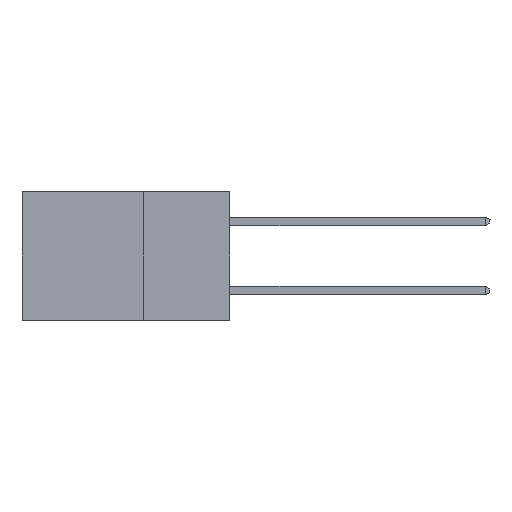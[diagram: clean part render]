
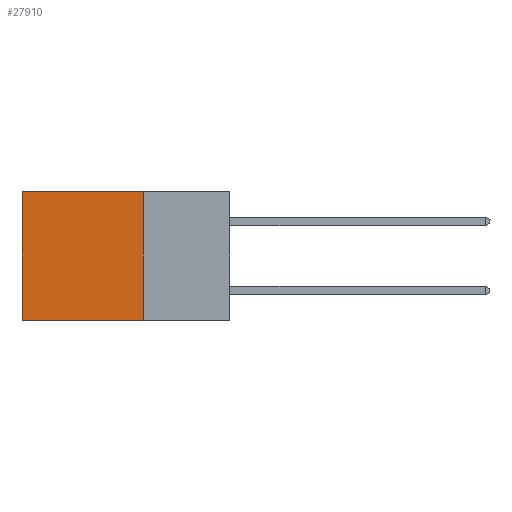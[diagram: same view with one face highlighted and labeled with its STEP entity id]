
A CAD part, left-side view. The second image highlights one B-rep face of the part: STEP entity #27910.
In plain terms, the highlighted planar face has unit normal (-1, 0, 0).
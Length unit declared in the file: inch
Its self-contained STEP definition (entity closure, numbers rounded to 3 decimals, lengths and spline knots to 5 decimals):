
#146 = VERTEX_POINT ( 'NONE', #16180 ) ;
#1535 = DIRECTION ( 'NONE',  ( 1., 0., 0. ) ) ;
#4924 = FACE_OUTER_BOUND ( 'NONE', #17492, .T. ) ;
#4960 = VECTOR ( 'NONE', #5991, 39.37008 ) ;
#5991 = DIRECTION ( 'NONE',  ( 0., 1., 0. ) ) ;
#7295 = DIRECTION ( 'NONE',  ( 0., 0., -1. ) ) ;
#7827 = CARTESIAN_POINT ( 'NONE',  ( 0.298, 0.6, 0. ) ) ;
#8591 = CARTESIAN_POINT ( 'NONE',  ( 0.298, 0.25, 0. ) ) ;
#10934 = CARTESIAN_POINT ( 'NONE',  ( 0.298, 0.25, -0.37 ) ) ;
#11558 = ORIENTED_EDGE ( 'NONE', *, *, #27721, .F. ) ;
#12032 = LINE ( 'NONE', #24882, #13230 ) ;
#12272 = VERTEX_POINT ( 'NONE', #10934 ) ;
#13230 = VECTOR ( 'NONE', #22468, 39.37008 ) ;
#13740 = VECTOR ( 'NONE', #7295, 39.37008 ) ;
#16180 = CARTESIAN_POINT ( 'NONE',  ( 0.298, 0.6, -0.37 ) ) ;
#16214 = EDGE_CURVE ( 'NONE', #20030, #17668, #18135, .T. ) ;
#16773 = PLANE ( 'NONE',  #28178 ) ;
#17492 = EDGE_LOOP ( 'NONE', ( #26882, #11558, #18700, #18011 ) ) ;
#17668 = VERTEX_POINT ( 'NONE', #7827 ) ;
#18011 = ORIENTED_EDGE ( 'NONE', *, *, #16214, .T. ) ;
#18135 = LINE ( 'NONE', #28933, #26448 ) ;
#18700 = ORIENTED_EDGE ( 'NONE', *, *, #28775, .F. ) ;
#19349 = DIRECTION ( 'NONE',  ( 0., 0., -1. ) ) ;
#19459 = CARTESIAN_POINT ( 'NONE',  ( 0.298, 0.25, 0. ) ) ;
#20030 = VERTEX_POINT ( 'NONE', #8591 ) ;
#20600 = LINE ( 'NONE', #23999, #4960 ) ;
#22468 = DIRECTION ( 'NONE',  ( 0., 0., -1. ) ) ;
#22736 = CARTESIAN_POINT ( 'NONE',  ( 0.298, 0.25, 0. ) ) ;
#23999 = CARTESIAN_POINT ( 'NONE',  ( 0.298, 0.25, -0.37 ) ) ;
#24882 = CARTESIAN_POINT ( 'NONE',  ( 0.298, 0.6, 0. ) ) ;
#24920 = EDGE_CURVE ( 'NONE', #17668, #146, #12032, .T. ) ;
#26448 = VECTOR ( 'NONE', #29152, 39.37008 ) ;
#26882 = ORIENTED_EDGE ( 'NONE', *, *, #24920, .T. ) ;
#27721 = EDGE_CURVE ( 'NONE', #12272, #146, #20600, .T. ) ;
#27910 = ADVANCED_FACE ( 'NONE', ( #4924 ), #16773, .F. ) ;
#28178 = AXIS2_PLACEMENT_3D ( 'NONE', #19459, #1535, #19349 ) ;
#28775 = EDGE_CURVE ( 'NONE', #20030, #12272, #32463, .T. ) ;
#28933 = CARTESIAN_POINT ( 'NONE',  ( 0.298, 0.25, 0. ) ) ;
#29152 = DIRECTION ( 'NONE',  ( 0., 1., 0. ) ) ;
#32463 = LINE ( 'NONE', #22736, #13740 ) ;
